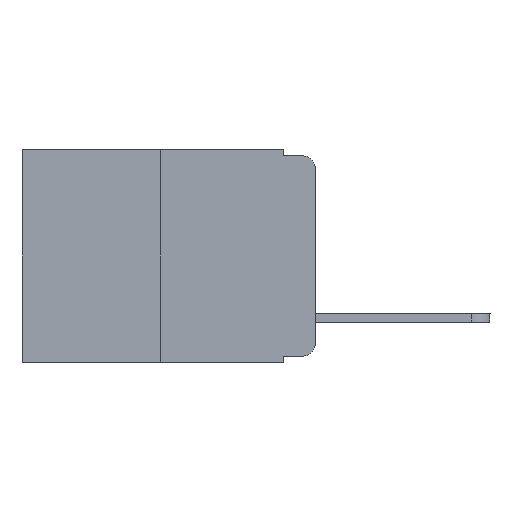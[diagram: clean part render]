
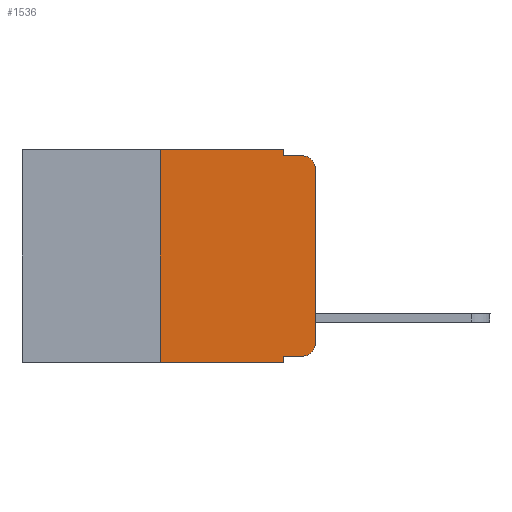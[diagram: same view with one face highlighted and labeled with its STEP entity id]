
A CAD part, left-side view. The second image highlights one B-rep face of the part: STEP entity #1536.
In plain terms, the highlighted planar face has unit normal (-1, 0, 0).
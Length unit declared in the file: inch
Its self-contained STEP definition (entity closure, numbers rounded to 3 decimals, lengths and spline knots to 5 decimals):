
#213 = CARTESIAN_POINT ( 'NONE',  ( 0., 0.02, -0.313 ) ) ;
#401 = CARTESIAN_POINT ( 'NONE',  ( 0., 0., 0. ) ) ;
#771 = DIRECTION ( 'NONE',  ( 0., 0., -1. ) ) ;
#1196 = ORIENTED_EDGE ( 'NONE', *, *, #19694, .F. ) ;
#1292 = DIRECTION ( 'NONE',  ( 0., 0., 1. ) ) ;
#1536 = ADVANCED_FACE ( 'NONE', ( #3735 ), #2377, .F. ) ;
#1684 = EDGE_CURVE ( 'NONE', #9150, #7995, #14959, .T. ) ;
#1878 = LINE ( 'NONE', #6304, #2447 ) ;
#1903 = LINE ( 'NONE', #401, #16801 ) ;
#2135 = DIRECTION ( 'NONE',  ( 0., -1., 0. ) ) ;
#2377 = PLANE ( 'NONE',  #22646 ) ;
#2447 = VECTOR ( 'NONE', #1292, 39.37008 ) ;
#2648 = VECTOR ( 'NONE', #22438, 39.37008 ) ;
#3156 = CARTESIAN_POINT ( 'NONE',  ( 0., 0., -0.03 ) ) ;
#3735 = FACE_OUTER_BOUND ( 'NONE', #9895, .T. ) ;
#4486 = CARTESIAN_POINT ( 'NONE',  ( 0., 0.051, 0. ) ) ;
#4488 = EDGE_CURVE ( 'NONE', #13237, #8328, #15446, .T. ) ;
#5114 = CARTESIAN_POINT ( 'NONE',  ( 0., 0.473, -0.343 ) ) ;
#5797 = CARTESIAN_POINT ( 'NONE',  ( 0., 0., -0.313 ) ) ;
#5992 = EDGE_CURVE ( 'NONE', #21757, #9150, #1878, .T. ) ;
#6304 = CARTESIAN_POINT ( 'NONE',  ( 0., 0.25, 0. ) ) ;
#6517 = VECTOR ( 'NONE', #13139, 39.37008 ) ;
#6715 = VECTOR ( 'NONE', #11252, 39.37008 ) ;
#7296 = LINE ( 'NONE', #18712, #16294 ) ;
#7349 = ORIENTED_EDGE ( 'NONE', *, *, #9697, .F. ) ;
#7613 = CARTESIAN_POINT ( 'NONE',  ( 0., 0.051, -0.333 ) ) ;
#7995 = VERTEX_POINT ( 'NONE', #4486 ) ;
#8328 = VERTEX_POINT ( 'NONE', #21545 ) ;
#8729 = CARTESIAN_POINT ( 'NONE',  ( 0., 0.02, -0.03 ) ) ;
#8886 = CARTESIAN_POINT ( 'NONE',  ( 0., 0.25, -0.343 ) ) ;
#8975 = ORIENTED_EDGE ( 'NONE', *, *, #12526, .T. ) ;
#9150 = VERTEX_POINT ( 'NONE', #18442 ) ;
#9425 = DIRECTION ( 'NONE',  ( 1., 0., 0. ) ) ;
#9452 = CARTESIAN_POINT ( 'NONE',  ( 0., 0.051, -0.343 ) ) ;
#9648 = ORIENTED_EDGE ( 'NONE', *, *, #4488, .T. ) ;
#9697 = EDGE_CURVE ( 'NONE', #12651, #19271, #22396, .T. ) ;
#9704 = EDGE_CURVE ( 'NONE', #13875, #17851, #1903, .T. ) ;
#9895 = EDGE_LOOP ( 'NONE', ( #16165, #12420, #7349, #1196, #21464, #15060, #20624, #16935, #9648, #8975 ) ) ;
#10189 = AXIS2_PLACEMENT_3D ( 'NONE', #8729, #15673, #12132 ) ;
#10209 = CARTESIAN_POINT ( 'NONE',  ( 0., 0.051, -0.333 ) ) ;
#10323 = CIRCLE ( 'NONE', #10189, 0.02 ) ;
#11100 = DIRECTION ( 'NONE',  ( 0., 0., 1. ) ) ;
#11210 = DIRECTION ( 'NONE',  ( -1., 0., 0. ) ) ;
#11252 = DIRECTION ( 'NONE',  ( 0., -1., 0. ) ) ;
#11641 = LINE ( 'NONE', #5114, #2648 ) ;
#11718 = DIRECTION ( 'NONE',  ( 0., 0., -1. ) ) ;
#11954 = CARTESIAN_POINT ( 'NONE',  ( 0., 0.051, 0. ) ) ;
#12132 = DIRECTION ( 'NONE',  ( 0., 0., -1. ) ) ;
#12420 = ORIENTED_EDGE ( 'NONE', *, *, #12867, .T. ) ;
#12526 = EDGE_CURVE ( 'NONE', #8328, #13875, #14833, .T. ) ;
#12578 = LINE ( 'NONE', #11954, #15111 ) ;
#12587 = CARTESIAN_POINT ( 'NONE',  ( 0., 0.02, -0.01 ) ) ;
#12651 = VERTEX_POINT ( 'NONE', #15426 ) ;
#12867 = EDGE_CURVE ( 'NONE', #17851, #19271, #10323, .T. ) ;
#12897 = DIRECTION ( 'NONE',  ( 0., 0., -1. ) ) ;
#13139 = DIRECTION ( 'NONE',  ( 0., -1., 0. ) ) ;
#13237 = VERTEX_POINT ( 'NONE', #7613 ) ;
#13875 = VERTEX_POINT ( 'NONE', #5797 ) ;
#14076 = CARTESIAN_POINT ( 'NONE',  ( 0., 0.473, 0. ) ) ;
#14833 = CIRCLE ( 'NONE', #16520, 0.02 ) ;
#14889 = EDGE_CURVE ( 'NONE', #21757, #18810, #11641, .T. ) ;
#14959 = LINE ( 'NONE', #14076, #6517 ) ;
#15060 = ORIENTED_EDGE ( 'NONE', *, *, #5992, .F. ) ;
#15111 = VECTOR ( 'NONE', #11718, 39.37008 ) ;
#15426 = CARTESIAN_POINT ( 'NONE',  ( 0., 0.051, -0.01 ) ) ;
#15446 = LINE ( 'NONE', #10209, #6715 ) ;
#15673 = DIRECTION ( 'NONE',  ( -1., 0., 0. ) ) ;
#16165 = ORIENTED_EDGE ( 'NONE', *, *, #9704, .T. ) ;
#16294 = VECTOR ( 'NONE', #771, 39.37008 ) ;
#16520 = AXIS2_PLACEMENT_3D ( 'NONE', #213, #11210, #20090 ) ;
#16576 = CARTESIAN_POINT ( 'NONE',  ( 0., 0.051, -0.01 ) ) ;
#16583 = CARTESIAN_POINT ( 'NONE',  ( 0., 0.473, 0. ) ) ;
#16801 = VECTOR ( 'NONE', #11100, 39.37008 ) ;
#16935 = ORIENTED_EDGE ( 'NONE', *, *, #17119, .F. ) ;
#17057 = VECTOR ( 'NONE', #2135, 39.37008 ) ;
#17119 = EDGE_CURVE ( 'NONE', #13237, #18810, #7296, .T. ) ;
#17851 = VERTEX_POINT ( 'NONE', #3156 ) ;
#18442 = CARTESIAN_POINT ( 'NONE',  ( 0., 0.25, 0. ) ) ;
#18712 = CARTESIAN_POINT ( 'NONE',  ( 0., 0.051, 0. ) ) ;
#18810 = VERTEX_POINT ( 'NONE', #9452 ) ;
#19271 = VERTEX_POINT ( 'NONE', #12587 ) ;
#19694 = EDGE_CURVE ( 'NONE', #7995, #12651, #12578, .T. ) ;
#20090 = DIRECTION ( 'NONE',  ( 0., 0., -1. ) ) ;
#20624 = ORIENTED_EDGE ( 'NONE', *, *, #14889, .T. ) ;
#21464 = ORIENTED_EDGE ( 'NONE', *, *, #1684, .F. ) ;
#21545 = CARTESIAN_POINT ( 'NONE',  ( 0., 0.02, -0.333 ) ) ;
#21757 = VERTEX_POINT ( 'NONE', #8886 ) ;
#22396 = LINE ( 'NONE', #16576, #17057 ) ;
#22438 = DIRECTION ( 'NONE',  ( 0., -1., 0. ) ) ;
#22646 = AXIS2_PLACEMENT_3D ( 'NONE', #16583, #9425, #12897 ) ;
